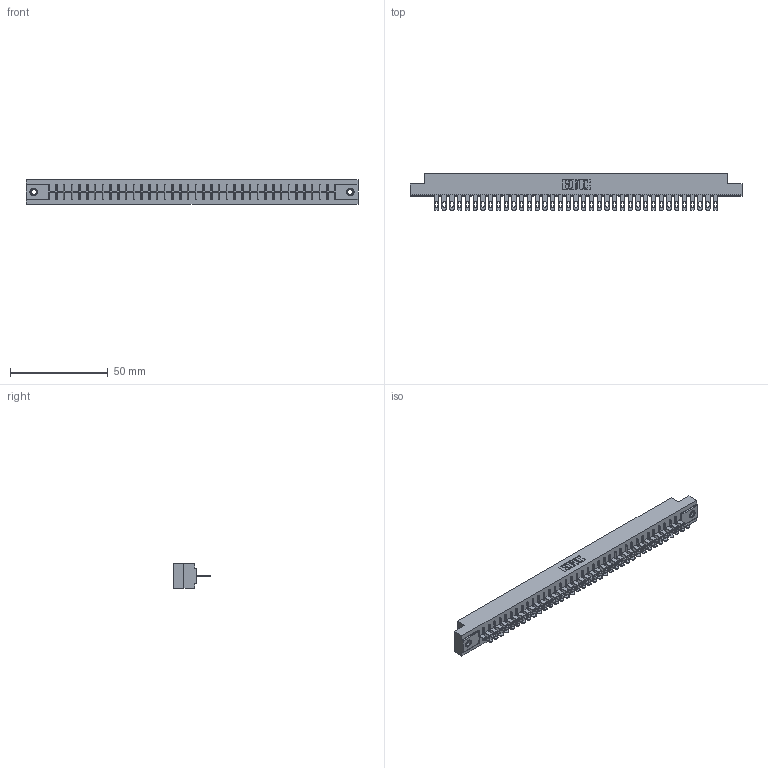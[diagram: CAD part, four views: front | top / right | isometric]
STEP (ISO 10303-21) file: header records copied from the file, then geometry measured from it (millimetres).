
FILE_DESCRIPTION (( 'STEP AP203' ), '1' );
FILE_NAME ('306-037-500-107.STEP', '2019-09-11T23:40:54', ( '' ), ( '' ), 'SwSTEP 2.0', 'SolidWorks 2016', '' );
FILE_SCHEMA (( 'CONFIG_CONTROL_DESIGN' ));
Length unit declared in the file: inch
Products named in the file (4): 306-290-001_100; 345-250-001_345-250-005-103; 306 Part_.156 Dia; 306-037-500-107
Assembly tree (40 placements, depth 2):
  306-037-500-107
    306 Part_.156 Dia
    306-290-001_100  x37
    345-250-001_345-250-005-103  x2
Bounding box: 169.62 x 18.87 x 12.7 mm (x, y, z)
Volume: 18817.1 mm3; surface area: 19949.3 mm2
Topology: 40 solids, 40 shells, 2988 faces, 8407 edges, 5398 vertices
Faces by surface type: plane 1950, cylinder 874, sphere 148, cone 12, torus 4
Entity records: 36501 total; most frequent: CARTESIAN_POINT 6109, ORIENTED_EDGE 6050, DIRECTION 6033, EDGE_CURVE 3025, VECTOR 2361, LINE 2361, VERTEX_POINT 1912, AXIS2_PLACEMENT_3D 1836
